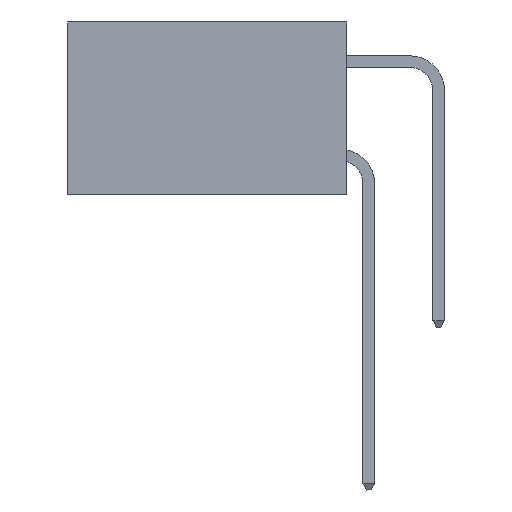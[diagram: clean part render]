
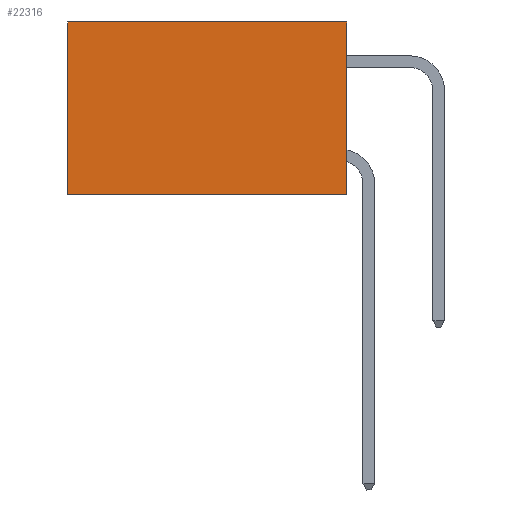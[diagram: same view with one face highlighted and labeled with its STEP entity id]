
A CAD part, left-side view. The second image highlights one B-rep face of the part: STEP entity #22316.
In plain terms, the highlighted planar face has unit normal (-1, 0, 0).
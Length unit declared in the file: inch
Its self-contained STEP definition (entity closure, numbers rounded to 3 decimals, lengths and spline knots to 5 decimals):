
#172 = FACE_OUTER_BOUND ( 'NONE', #11529, .T. ) ;
#224 = ORIENTED_EDGE ( 'NONE', *, *, #18350, .T. ) ;
#1656 = VECTOR ( 'NONE', #10670, 39.37008 ) ;
#1919 = DIRECTION ( 'NONE',  ( 0., 1., 0. ) ) ;
#1994 = CARTESIAN_POINT ( 'NONE',  ( 0.2875, 0., -0.37 ) ) ;
#4211 = PLANE ( 'NONE',  #15219 ) ;
#5074 = LINE ( 'NONE', #16520, #18240 ) ;
#5260 = CARTESIAN_POINT ( 'NONE',  ( 0.2875, 0., 0. ) ) ;
#6336 = CARTESIAN_POINT ( 'NONE',  ( 0.2875, 0.6, 0. ) ) ;
#7075 = EDGE_CURVE ( 'NONE', #14218, #20250, #5074, .T. ) ;
#7833 = DIRECTION ( 'NONE',  ( 1., 0., 0. ) ) ;
#8375 = VERTEX_POINT ( 'NONE', #9651 ) ;
#8900 = EDGE_CURVE ( 'NONE', #8375, #10135, #22572, .T. ) ;
#9313 = DIRECTION ( 'NONE',  ( 0., 1., 0. ) ) ;
#9651 = CARTESIAN_POINT ( 'NONE',  ( 0.2875, 0., -0.37 ) ) ;
#10135 = VERTEX_POINT ( 'NONE', #20075 ) ;
#10670 = DIRECTION ( 'NONE',  ( 0., 0., -1. ) ) ;
#11529 = EDGE_LOOP ( 'NONE', ( #224, #17093, #14221, #22007 ) ) ;
#12291 = CARTESIAN_POINT ( 'NONE',  ( 0.2875, 0.6, 0. ) ) ;
#12594 = VECTOR ( 'NONE', #1919, 39.37008 ) ;
#13981 = EDGE_CURVE ( 'NONE', #14218, #8375, #15996, .T. ) ;
#14076 = DIRECTION ( 'NONE',  ( 0., 0., -1. ) ) ;
#14218 = VERTEX_POINT ( 'NONE', #14817 ) ;
#14221 = ORIENTED_EDGE ( 'NONE', *, *, #13981, .F. ) ;
#14424 = VECTOR ( 'NONE', #14076, 39.37008 ) ;
#14817 = CARTESIAN_POINT ( 'NONE',  ( 0.2875, 0., 0. ) ) ;
#14961 = CARTESIAN_POINT ( 'NONE',  ( 0.2875, 0., 0. ) ) ;
#15219 = AXIS2_PLACEMENT_3D ( 'NONE', #14961, #7833, #20301 ) ;
#15996 = LINE ( 'NONE', #5260, #1656 ) ;
#16520 = CARTESIAN_POINT ( 'NONE',  ( 0.2875, 0., 0. ) ) ;
#17093 = ORIENTED_EDGE ( 'NONE', *, *, #8900, .F. ) ;
#18240 = VECTOR ( 'NONE', #9313, 39.37008 ) ;
#18350 = EDGE_CURVE ( 'NONE', #20250, #10135, #19130, .T. ) ;
#19130 = LINE ( 'NONE', #12291, #14424 ) ;
#20075 = CARTESIAN_POINT ( 'NONE',  ( 0.2875, 0.6, -0.37 ) ) ;
#20250 = VERTEX_POINT ( 'NONE', #6336 ) ;
#20301 = DIRECTION ( 'NONE',  ( 0., 0., -1. ) ) ;
#22007 = ORIENTED_EDGE ( 'NONE', *, *, #7075, .T. ) ;
#22316 = ADVANCED_FACE ( 'NONE', ( #172 ), #4211, .F. ) ;
#22572 = LINE ( 'NONE', #1994, #12594 ) ;
